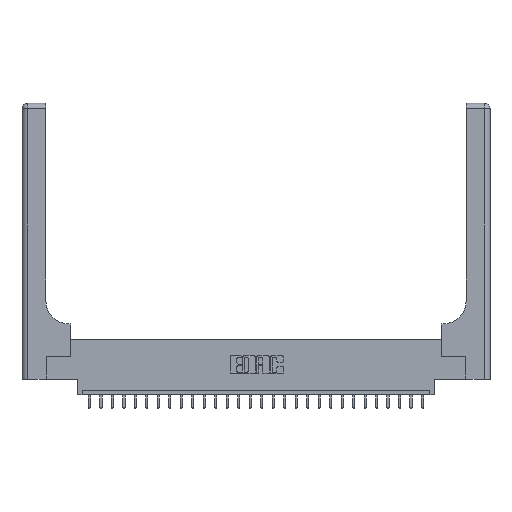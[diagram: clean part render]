
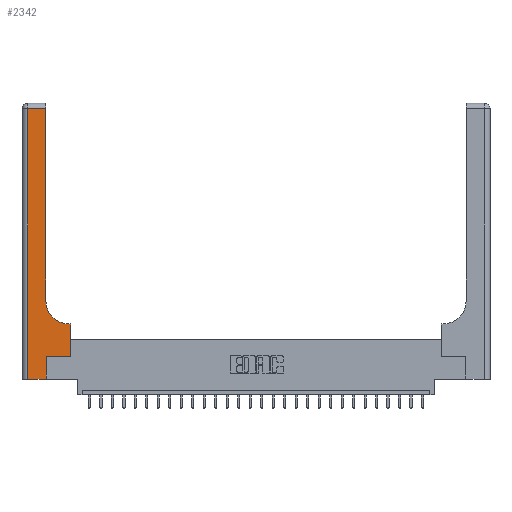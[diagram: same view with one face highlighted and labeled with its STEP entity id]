
A CAD part, top view. The second image highlights one B-rep face of the part: STEP entity #2342.
In plain terms, the highlighted planar face has unit normal (0, 0, 1).
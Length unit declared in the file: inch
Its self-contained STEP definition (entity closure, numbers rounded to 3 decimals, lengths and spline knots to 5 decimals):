
#280 = DIRECTION ( 'NONE',  ( -1., 0., 0. ) ) ;
#326 = CARTESIAN_POINT ( 'NONE',  ( 0.26, 3., 0.37 ) ) ;
#1294 = CARTESIAN_POINT ( 'NONE',  ( 0.51, 0.85, 0.37 ) ) ;
#1602 = VECTOR ( 'NONE', #24939, 39.37008 ) ;
#2058 = ORIENTED_EDGE ( 'NONE', *, *, #11461, .T. ) ;
#2342 = ADVANCED_FACE ( 'NONE', ( #5608 ), #19899, .F. ) ;
#2494 = DIRECTION ( 'NONE',  ( 0., 1., 0. ) ) ;
#2905 = VECTOR ( 'NONE', #9160, 39.37008 ) ;
#3516 = LINE ( 'NONE', #12677, #14607 ) ;
#3662 = CARTESIAN_POINT ( 'NONE',  ( 0.51, 0.6, 0.37 ) ) ;
#3733 = CARTESIAN_POINT ( 'NONE',  ( 0.26, 2.94, 0.37 ) ) ;
#4021 = VERTEX_POINT ( 'NONE', #3733 ) ;
#4142 = ORIENTED_EDGE ( 'NONE', *, *, #8071, .T. ) ;
#4935 = AXIS2_PLACEMENT_3D ( 'NONE', #1294, #16967, #15110 ) ;
#5003 = VERTEX_POINT ( 'NONE', #6692 ) ;
#5351 = VECTOR ( 'NONE', #13325, 39.37008 ) ;
#5608 = FACE_OUTER_BOUND ( 'NONE', #15788, .T. ) ;
#6042 = VECTOR ( 'NONE', #12163, 39.37008 ) ;
#6326 = CARTESIAN_POINT ( 'NONE',  ( 0., 3., 0.37 ) ) ;
#6692 = CARTESIAN_POINT ( 'NONE',  ( 0.265, 0.25, 0.37 ) ) ;
#7286 = ORIENTED_EDGE ( 'NONE', *, *, #7712, .T. ) ;
#7431 = CARTESIAN_POINT ( 'NONE',  ( 0.06, 2.94, 0.37 ) ) ;
#7447 = EDGE_CURVE ( 'NONE', #10851, #17090, #16150, .T. ) ;
#7712 = EDGE_CURVE ( 'NONE', #17090, #8345, #3516, .T. ) ;
#7868 = VERTEX_POINT ( 'NONE', #3662 ) ;
#7912 = EDGE_CURVE ( 'NONE', #13280, #7868, #13672, .T. ) ;
#8071 = EDGE_CURVE ( 'NONE', #8445, #13280, #17035, .T. ) ;
#8174 = EDGE_CURVE ( 'NONE', #4021, #10851, #20386, .T. ) ;
#8345 = VERTEX_POINT ( 'NONE', #16252 ) ;
#8445 = VERTEX_POINT ( 'NONE', #20094 ) ;
#9160 = DIRECTION ( 'NONE',  ( 0., -1., 0. ) ) ;
#10257 = CIRCLE ( 'NONE', #4935, 0.25 ) ;
#10851 = VERTEX_POINT ( 'NONE', #7431 ) ;
#11031 = DIRECTION ( 'NONE',  ( 1., 0., 0. ) ) ;
#11461 = EDGE_CURVE ( 'NONE', #8345, #5003, #11898, .T. ) ;
#11480 = CARTESIAN_POINT ( 'NONE',  ( 0.265, 0.25, 0.37 ) ) ;
#11897 = CARTESIAN_POINT ( 'NONE',  ( 0.26, 0.6, 0.37 ) ) ;
#11898 = LINE ( 'NONE', #12253, #6042 ) ;
#12163 = DIRECTION ( 'NONE',  ( 0., 1., 0. ) ) ;
#12238 = VERTEX_POINT ( 'NONE', #19833 ) ;
#12253 = CARTESIAN_POINT ( 'NONE',  ( 0.265, 0., 0.37 ) ) ;
#12677 = CARTESIAN_POINT ( 'NONE',  ( 0., 0., 0.37 ) ) ;
#12777 = DIRECTION ( 'NONE',  ( -1., 0., 0. ) ) ;
#13280 = VERTEX_POINT ( 'NONE', #17906 ) ;
#13325 = DIRECTION ( 'NONE',  ( 0., 1., 0. ) ) ;
#13423 = EDGE_CURVE ( 'NONE', #7868, #12238, #10257, .T. ) ;
#13580 = ORIENTED_EDGE ( 'NONE', *, *, #18549, .T. ) ;
#13672 = LINE ( 'NONE', #11897, #17950 ) ;
#14405 = CARTESIAN_POINT ( 'NONE',  ( 0., 2.94, 0.37 ) ) ;
#14574 = LINE ( 'NONE', #11480, #1602 ) ;
#14607 = VECTOR ( 'NONE', #11031, 39.37008 ) ;
#15110 = DIRECTION ( 'NONE',  ( 1., 0., 0. ) ) ;
#15788 = EDGE_LOOP ( 'NONE', ( #13580, #24133, #25499, #7286, #2058, #24472, #4142, #21029, #19638 ) ) ;
#16150 = LINE ( 'NONE', #22200, #2905 ) ;
#16252 = CARTESIAN_POINT ( 'NONE',  ( 0.265, 0., 0.37 ) ) ;
#16326 = DIRECTION ( 'NONE',  ( 0., 0., -1. ) ) ;
#16967 = DIRECTION ( 'NONE',  ( 0., 0., -1. ) ) ;
#17035 = LINE ( 'NONE', #23293, #5351 ) ;
#17037 = CARTESIAN_POINT ( 'NONE',  ( 0.06, 0., 0.37 ) ) ;
#17090 = VERTEX_POINT ( 'NONE', #17037 ) ;
#17906 = CARTESIAN_POINT ( 'NONE',  ( 0.528, 0.6, 0.37 ) ) ;
#17950 = VECTOR ( 'NONE', #23804, 39.37008 ) ;
#18549 = EDGE_CURVE ( 'NONE', #12238, #4021, #19611, .T. ) ;
#19611 = LINE ( 'NONE', #326, #24632 ) ;
#19638 = ORIENTED_EDGE ( 'NONE', *, *, #13423, .T. ) ;
#19833 = CARTESIAN_POINT ( 'NONE',  ( 0.26, 0.85, 0.37 ) ) ;
#19899 = PLANE ( 'NONE',  #22914 ) ;
#20094 = CARTESIAN_POINT ( 'NONE',  ( 0.528, 0.25, 0.37 ) ) ;
#20386 = LINE ( 'NONE', #14405, #21900 ) ;
#21029 = ORIENTED_EDGE ( 'NONE', *, *, #7912, .T. ) ;
#21900 = VECTOR ( 'NONE', #12777, 39.37008 ) ;
#22200 = CARTESIAN_POINT ( 'NONE',  ( 0.06, 3., 0.37 ) ) ;
#22914 = AXIS2_PLACEMENT_3D ( 'NONE', #6326, #16326, #280 ) ;
#23293 = CARTESIAN_POINT ( 'NONE',  ( 0.528, 0.25, 0.37 ) ) ;
#23804 = DIRECTION ( 'NONE',  ( -1., 0., 0. ) ) ;
#24133 = ORIENTED_EDGE ( 'NONE', *, *, #8174, .T. ) ;
#24472 = ORIENTED_EDGE ( 'NONE', *, *, #25092, .T. ) ;
#24632 = VECTOR ( 'NONE', #2494, 39.37008 ) ;
#24939 = DIRECTION ( 'NONE',  ( 1., 0., 0. ) ) ;
#25092 = EDGE_CURVE ( 'NONE', #5003, #8445, #14574, .T. ) ;
#25499 = ORIENTED_EDGE ( 'NONE', *, *, #7447, .T. ) ;
